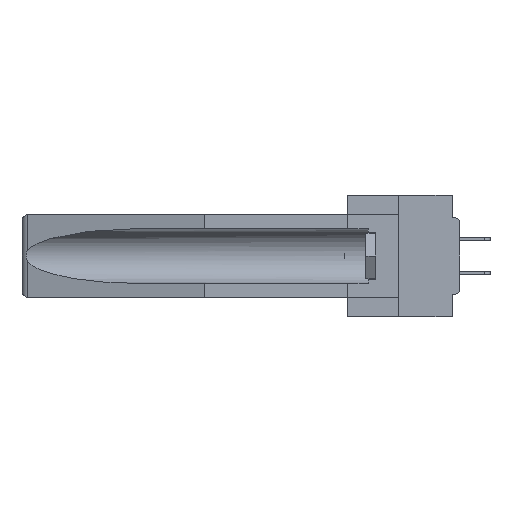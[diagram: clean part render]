
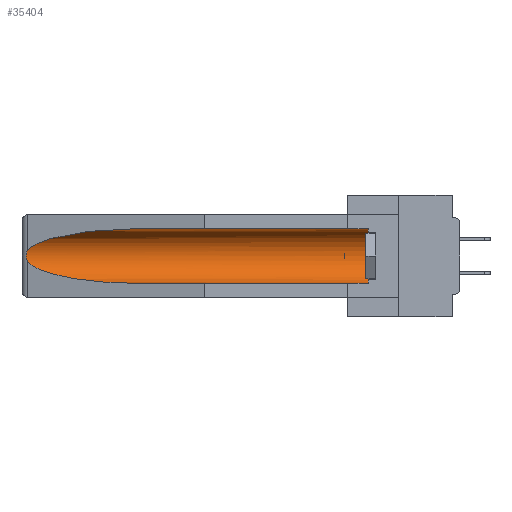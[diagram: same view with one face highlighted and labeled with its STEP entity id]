
A CAD part, left-side view. The second image highlights one B-rep face of the part: STEP entity #35404.
In plain terms, the highlighted cylindrical face has radius 2.857 mm (diameter 5.715 mm), a partial arc.
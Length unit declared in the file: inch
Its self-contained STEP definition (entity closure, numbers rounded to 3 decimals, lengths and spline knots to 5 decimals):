
#175 = ORIENTED_EDGE ( 'NONE', *, *, #4700, .T. ) ;
#1538 = DIRECTION ( 'NONE',  ( 0., 1., 0. ) ) ;
#1627 = CARTESIAN_POINT ( 'NONE',  ( 0.155, 0.126, -0.284 ) ) ;
#4700 = EDGE_CURVE ( 'NONE', #35125, #36528, #47589, .T. ) ;
#5000 = EDGE_CURVE ( 'NONE', #26393, #26674, #17092, .T. ) ;
#7713 = FACE_OUTER_BOUND ( 'NONE', #32933, .T. ) ;
#9177 = EDGE_CURVE ( 'NONE', #23017, #46629, #46894, .T. ) ;
#9448 = CYLINDRICAL_SURFACE ( 'NONE', #42875, 0.1125 ) ;
#9657 = CARTESIAN_POINT ( 'NONE',  ( 0.26537, 1.52718, -0.19328 ) ) ;
#9790 = CARTESIAN_POINT ( 'NONE',  ( 0.155, 1.07973, -0.059 ) ) ;
#10642 = ORIENTED_EDGE ( 'NONE', *, *, #24271, .T. ) ;
#13328 = VECTOR ( 'NONE', #35542, 39.37008 ) ;
#13406 = CARTESIAN_POINT ( 'NONE',  ( 0.26537, 1.52718, -0.14972 ) ) ;
#14345 = CARTESIAN_POINT ( 'NONE',  ( 0.155, 0.126, -0.1715 ) ) ;
#15270 = AXIS2_PLACEMENT_3D ( 'NONE', #14345, #17956, #40682 ) ;
#15509 = EDGE_CURVE ( 'NONE', #36528, #46629, #46703, .T. ) ;
#17092 = LINE ( 'NONE', #40561, #25963 ) ;
#17956 = DIRECTION ( 'NONE',  ( 0., -1., 0. ) ) ;
#18612 = ORIENTED_EDGE ( 'NONE', *, *, #9177, .F. ) ;
#20537 = CARTESIAN_POINT ( 'NONE',  ( 0.155, 1.07973, -0.284 ) ) ;
#20816 = CARTESIAN_POINT ( 'NONE',  ( 0.26597, 1.5296, -0.19026 ) ) ;
#20977 = CARTESIAN_POINT ( 'NONE',  ( 0.26654, 1.53092, -0.15636 ) ) ;
#21341 =( BOUNDED_CURVE ( )  B_SPLINE_CURVE ( 3, ( #9790, #36128, #47473, #13406 ),
 .UNSPECIFIED., .F., .T. ) 
 B_SPLINE_CURVE_WITH_KNOTS ( ( 4, 4 ),
 ( 4.71239, 6.08839 ),
 .UNSPECIFIED. ) 
 CURVE ( )  GEOMETRIC_REPRESENTATION_ITEM ( )  RATIONAL_B_SPLINE_CURVE ( ( 1., 0.848, 0.848, 1. ) ) 
 REPRESENTATION_ITEM ( '' )  );
#23017 = VERTEX_POINT ( 'NONE', #1627 ) ;
#24271 = EDGE_CURVE ( 'NONE', #26674, #35125, #21341, .T. ) ;
#24962 = CARTESIAN_POINT ( 'NONE',  ( 0.2675, 1.53308, -0.17534 ) ) ;
#25117 = CARTESIAN_POINT ( 'NONE',  ( 0.2673, 1.53269, -0.17917 ) ) ;
#25963 = VECTOR ( 'NONE', #36773, 39.37008 ) ;
#26081 = EDGE_CURVE ( 'NONE', #23017, #26393, #35653, .T. ) ;
#26393 = VERTEX_POINT ( 'NONE', #30585 ) ;
#26674 = VERTEX_POINT ( 'NONE', #33686 ) ;
#26690 = ORIENTED_EDGE ( 'NONE', *, *, #5000, .T. ) ;
#27123 = ORIENTED_EDGE ( 'NONE', *, *, #26081, .T. ) ;
#28384 = CARTESIAN_POINT ( 'NONE',  ( 0.2673, 1.5327, -0.16383 ) ) ;
#28748 = CARTESIAN_POINT ( 'NONE',  ( 0.25451, 1.48313, -0.24835 ) ) ;
#30585 = CARTESIAN_POINT ( 'NONE',  ( 0.155, 0.126, -0.059 ) ) ;
#32210 = CARTESIAN_POINT ( 'NONE',  ( 0.26537, 1.52718, -0.19328 ) ) ;
#32372 = CARTESIAN_POINT ( 'NONE',  ( 0.26597, 1.52961, -0.15275 ) ) ;
#32690 = CARTESIAN_POINT ( 'NONE',  ( 0.26537, 1.52718, -0.14972 ) ) ;
#32933 = EDGE_LOOP ( 'NONE', ( #10642, #175, #34357, #18612, #27123, #26690 ) ) ;
#33686 = CARTESIAN_POINT ( 'NONE',  ( 0.155, 1.07973, -0.059 ) ) ;
#34357 = ORIENTED_EDGE ( 'NONE', *, *, #15509, .T. ) ;
#34416 = CARTESIAN_POINT ( 'NONE',  ( 0.26537, 1.52718, -0.14972 ) ) ;
#35125 = VERTEX_POINT ( 'NONE', #34416 ) ;
#35404 = ADVANCED_FACE ( 'NONE', ( #7713 ), #9448, .F. ) ;
#35542 = DIRECTION ( 'NONE',  ( 0., 1., 0. ) ) ;
#35653 = CIRCLE ( 'NONE', #15270, 0.1125 ) ;
#35810 = CARTESIAN_POINT ( 'NONE',  ( 0.26655, 1.53094, -0.18657 ) ) ;
#35860 = CARTESIAN_POINT ( 'NONE',  ( 0.155, -0.30754, -0.284 ) ) ;
#36128 = CARTESIAN_POINT ( 'NONE',  ( 0.21114, 1.30732, -0.059 ) ) ;
#36259 = CARTESIAN_POINT ( 'NONE',  ( 0.2675, 1.53308, -0.16763 ) ) ;
#36528 = VERTEX_POINT ( 'NONE', #47784 ) ;
#36773 = DIRECTION ( 'NONE',  ( 0., 1., 0. ) ) ;
#40561 = CARTESIAN_POINT ( 'NONE',  ( 0.155, -0.30754, -0.059 ) ) ;
#40682 = DIRECTION ( 'NONE',  ( 0., 0., 1. ) ) ;
#42875 = AXIS2_PLACEMENT_3D ( 'NONE', #46775, #1538, #43485 ) ;
#43090 = CARTESIAN_POINT ( 'NONE',  ( 0.155, 1.07973, -0.284 ) ) ;
#43485 = DIRECTION ( 'NONE',  ( 0., 0., 1. ) ) ;
#46629 = VERTEX_POINT ( 'NONE', #43090 ) ;
#46703 =( BOUNDED_CURVE ( )  B_SPLINE_CURVE ( 3, ( #9657, #28748, #47177, #20537 ),
 .UNSPECIFIED., .F., .F. ) 
 B_SPLINE_CURVE_WITH_KNOTS ( ( 4, 4 ),
 ( 0.1948, 1.5708 ),
 .UNSPECIFIED. ) 
 CURVE ( )  GEOMETRIC_REPRESENTATION_ITEM ( )  RATIONAL_B_SPLINE_CURVE ( ( 1., 0.848, 0.848, 1. ) ) 
 REPRESENTATION_ITEM ( '' )  );
#46775 = CARTESIAN_POINT ( 'NONE',  ( 0.155, -0.30754, -0.1715 ) ) ;
#46894 = LINE ( 'NONE', #35860, #13328 ) ;
#47177 = CARTESIAN_POINT ( 'NONE',  ( 0.21114, 1.30732, -0.284 ) ) ;
#47473 = CARTESIAN_POINT ( 'NONE',  ( 0.25451, 1.48313, -0.09465 ) ) ;
#47589 = B_SPLINE_CURVE_WITH_KNOTS ( 'NONE', 3,
 ( #32690, #32372, #20977, #28384, #36259, #24962, #25117, #35810, #20816, #32210 ),
 .UNSPECIFIED., .F., .F.,
 ( 4, 2, 2, 2, 4 ),
 ( 0., 0.00029, 0.00058, 0.00087, 0.00117 ),
 .UNSPECIFIED. ) ;
#47784 = CARTESIAN_POINT ( 'NONE',  ( 0.26537, 1.52718, -0.19328 ) ) ;
